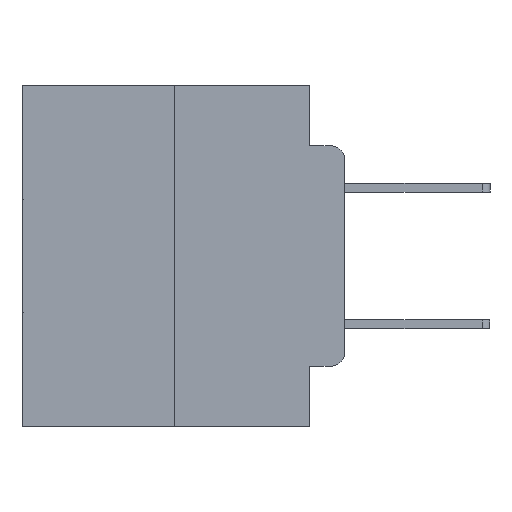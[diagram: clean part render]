
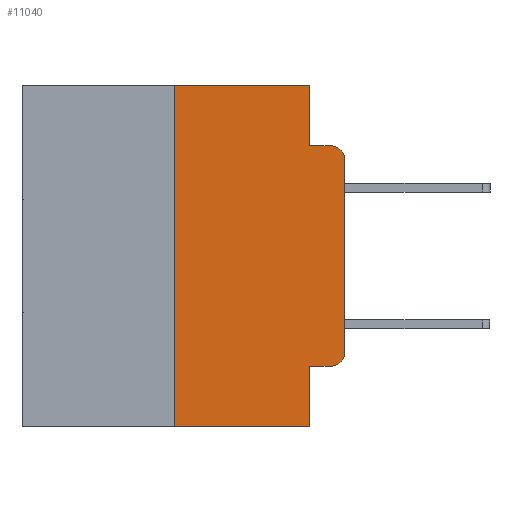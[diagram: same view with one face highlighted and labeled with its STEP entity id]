
A CAD part, left-side view. The second image highlights one B-rep face of the part: STEP entity #11040.
In plain terms, the highlighted planar face has unit normal (-1, 0, 0).
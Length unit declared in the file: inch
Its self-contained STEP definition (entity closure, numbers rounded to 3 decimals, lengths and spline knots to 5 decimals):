
#383 = EDGE_CURVE ( 'NONE', #13060, #20644, #13513, .T. ) ;
#395 = CARTESIAN_POINT ( 'NONE',  ( 0., 0.051, 0. ) ) ;
#616 = CARTESIAN_POINT ( 'NONE',  ( 0., 0.051, -0.5 ) ) ;
#1467 = EDGE_CURVE ( 'NONE', #13217, #13443, #5525, .T. ) ;
#1561 = CARTESIAN_POINT ( 'NONE',  ( 0., 0.051, -0.0885 ) ) ;
#2109 = AXIS2_PLACEMENT_3D ( 'NONE', #12861, #27751, #15071 ) ;
#2897 = ORIENTED_EDGE ( 'NONE', *, *, #1467, .F. ) ;
#3155 = LINE ( 'NONE', #12217, #25531 ) ;
#3198 = CIRCLE ( 'NONE', #12575, 0.02 ) ;
#3599 = ORIENTED_EDGE ( 'NONE', *, *, #13947, .T. ) ;
#3606 = CARTESIAN_POINT ( 'NONE',  ( 0., 0.051, -0.4115 ) ) ;
#3616 = EDGE_CURVE ( 'NONE', #17071, #26902, #4640, .T. ) ;
#3955 = VECTOR ( 'NONE', #22209, 39.37008 ) ;
#4000 = CARTESIAN_POINT ( 'NONE',  ( 0., 0.02, -0.0885 ) ) ;
#4566 = EDGE_CURVE ( 'NONE', #15993, #20644, #3155, .T. ) ;
#4640 = LINE ( 'NONE', #4834, #3955 ) ;
#4794 = VERTEX_POINT ( 'NONE', #15211 ) ;
#4834 = CARTESIAN_POINT ( 'NONE',  ( 0., 0., 0. ) ) ;
#5470 = PLANE ( 'NONE',  #22240 ) ;
#5525 = LINE ( 'NONE', #8922, #15827 ) ;
#5824 = ORIENTED_EDGE ( 'NONE', *, *, #26783, .F. ) ;
#6034 = VERTEX_POINT ( 'NONE', #4000 ) ;
#8077 = CARTESIAN_POINT ( 'NONE',  ( 0., 0.25, -0.5 ) ) ;
#8575 = CARTESIAN_POINT ( 'NONE',  ( 0., 0.25, 0. ) ) ;
#8714 = DIRECTION ( 'NONE',  ( 0., 0., 1. ) ) ;
#8835 = ORIENTED_EDGE ( 'NONE', *, *, #3616, .T. ) ;
#8922 = CARTESIAN_POINT ( 'NONE',  ( 0., 0.473, 0. ) ) ;
#9618 = VECTOR ( 'NONE', #14816, 39.37008 ) ;
#9739 = CARTESIAN_POINT ( 'NONE',  ( 0., 0.02, -0.1085 ) ) ;
#9774 = DIRECTION ( 'NONE',  ( 0., 0., -1. ) ) ;
#9917 = CARTESIAN_POINT ( 'NONE',  ( 0., 0.473, 0. ) ) ;
#10645 = VECTOR ( 'NONE', #9774, 39.37008 ) ;
#10964 = ORIENTED_EDGE ( 'NONE', *, *, #17569, .T. ) ;
#11040 = ADVANCED_FACE ( 'NONE', ( #24493 ), #5470, .F. ) ;
#11320 = VECTOR ( 'NONE', #8714, 39.37008 ) ;
#11958 = ORIENTED_EDGE ( 'NONE', *, *, #14698, .T. ) ;
#11968 = DIRECTION ( 'NONE',  ( 0., 0., -1. ) ) ;
#12138 = DIRECTION ( 'NONE',  ( 0., 0., -1. ) ) ;
#12217 = CARTESIAN_POINT ( 'NONE',  ( 0., 0.051, 0. ) ) ;
#12439 = DIRECTION ( 'NONE',  ( 0., -1., 0. ) ) ;
#12487 = EDGE_CURVE ( 'NONE', #4794, #6034, #21118, .T. ) ;
#12575 = AXIS2_PLACEMENT_3D ( 'NONE', #9739, #24768, #11968 ) ;
#12861 = CARTESIAN_POINT ( 'NONE',  ( 0., 0.02, -0.3915 ) ) ;
#12895 = CARTESIAN_POINT ( 'NONE',  ( 0., 0.02, -0.4115 ) ) ;
#12925 = CARTESIAN_POINT ( 'NONE',  ( 0., 0.25, 0. ) ) ;
#13060 = VERTEX_POINT ( 'NONE', #8077 ) ;
#13217 = VERTEX_POINT ( 'NONE', #8575 ) ;
#13408 = ORIENTED_EDGE ( 'NONE', *, *, #4566, .F. ) ;
#13443 = VERTEX_POINT ( 'NONE', #395 ) ;
#13513 = LINE ( 'NONE', #15645, #24199 ) ;
#13878 = EDGE_LOOP ( 'NONE', ( #8835, #3599, #17013, #5824, #2897, #26392, #15898, #13408, #11958, #10964 ) ) ;
#13947 = EDGE_CURVE ( 'NONE', #26902, #6034, #3198, .T. ) ;
#14698 = EDGE_CURVE ( 'NONE', #15993, #25625, #22573, .T. ) ;
#14816 = DIRECTION ( 'NONE',  ( 0., -1., 0. ) ) ;
#14851 = CARTESIAN_POINT ( 'NONE',  ( 0., 0., -0.1085 ) ) ;
#15071 = DIRECTION ( 'NONE',  ( 0., 0., -1. ) ) ;
#15211 = CARTESIAN_POINT ( 'NONE',  ( 0., 0.051, -0.0885 ) ) ;
#15560 = CARTESIAN_POINT ( 'NONE',  ( 0., 0., -0.3915 ) ) ;
#15645 = CARTESIAN_POINT ( 'NONE',  ( 0., 0.473, -0.5 ) ) ;
#15827 = VECTOR ( 'NONE', #12439, 39.37008 ) ;
#15898 = ORIENTED_EDGE ( 'NONE', *, *, #383, .T. ) ;
#15993 = VERTEX_POINT ( 'NONE', #23396 ) ;
#16714 = DIRECTION ( 'NONE',  ( 0., -1., 0. ) ) ;
#16883 = VECTOR ( 'NONE', #16714, 39.37008 ) ;
#17013 = ORIENTED_EDGE ( 'NONE', *, *, #12487, .F. ) ;
#17071 = VERTEX_POINT ( 'NONE', #15560 ) ;
#17569 = EDGE_CURVE ( 'NONE', #25625, #17071, #18092, .T. ) ;
#18092 = CIRCLE ( 'NONE', #2109, 0.02 ) ;
#18256 = EDGE_CURVE ( 'NONE', #13060, #13217, #22744, .T. ) ;
#18381 = CARTESIAN_POINT ( 'NONE',  ( 0., 0.051, 0. ) ) ;
#20644 = VERTEX_POINT ( 'NONE', #616 ) ;
#21118 = LINE ( 'NONE', #1561, #9618 ) ;
#22209 = DIRECTION ( 'NONE',  ( 0., 0., 1. ) ) ;
#22240 = AXIS2_PLACEMENT_3D ( 'NONE', #9917, #24928, #12138 ) ;
#22573 = LINE ( 'NONE', #3606, #16883 ) ;
#22744 = LINE ( 'NONE', #12925, #11320 ) ;
#22899 = DIRECTION ( 'NONE',  ( 0., 0., -1. ) ) ;
#23396 = CARTESIAN_POINT ( 'NONE',  ( 0., 0.051, -0.4115 ) ) ;
#24199 = VECTOR ( 'NONE', #25802, 39.37008 ) ;
#24493 = FACE_OUTER_BOUND ( 'NONE', #13878, .T. ) ;
#24768 = DIRECTION ( 'NONE',  ( -1., 0., 0. ) ) ;
#24928 = DIRECTION ( 'NONE',  ( 1., 0., 0. ) ) ;
#25531 = VECTOR ( 'NONE', #22899, 39.37008 ) ;
#25625 = VERTEX_POINT ( 'NONE', #12895 ) ;
#25802 = DIRECTION ( 'NONE',  ( 0., -1., 0. ) ) ;
#26392 = ORIENTED_EDGE ( 'NONE', *, *, #18256, .F. ) ;
#26783 = EDGE_CURVE ( 'NONE', #13443, #4794, #27039, .T. ) ;
#26902 = VERTEX_POINT ( 'NONE', #14851 ) ;
#27039 = LINE ( 'NONE', #18381, #10645 ) ;
#27751 = DIRECTION ( 'NONE',  ( -1., 0., 0. ) ) ;
